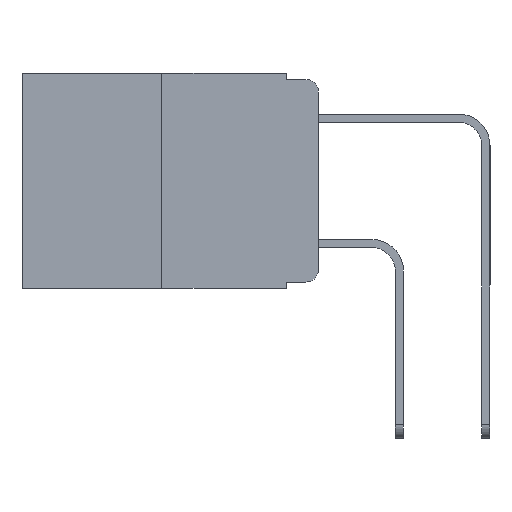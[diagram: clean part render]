
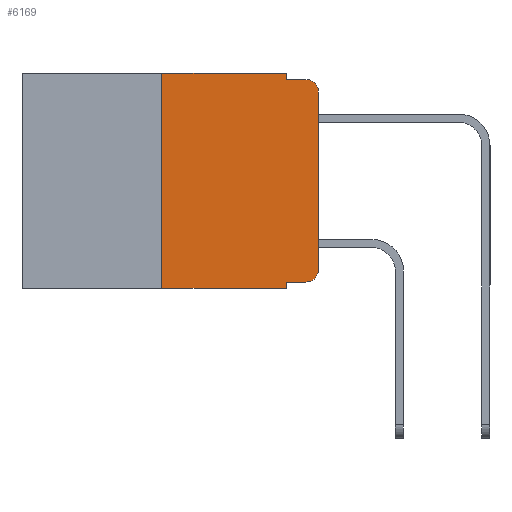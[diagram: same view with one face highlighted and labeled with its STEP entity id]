
A CAD part, left-side view. The second image highlights one B-rep face of the part: STEP entity #6169.
In plain terms, the highlighted planar face has unit normal (-1, 0, 0).
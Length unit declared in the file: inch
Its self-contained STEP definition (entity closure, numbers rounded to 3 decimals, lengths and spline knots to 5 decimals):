
#873 = VECTOR ( 'NONE', #3236, 39.37008 ) ;
#1132 = CARTESIAN_POINT ( 'NONE',  ( 0., 0.02, -0.313 ) ) ;
#1244 = EDGE_CURVE ( 'NONE', #6754, #8812, #8413, .T. ) ;
#1344 = ORIENTED_EDGE ( 'NONE', *, *, #3674, .T. ) ;
#1407 = ORIENTED_EDGE ( 'NONE', *, *, #5270, .T. ) ;
#1428 = ORIENTED_EDGE ( 'NONE', *, *, #2889, .F. ) ;
#1588 = ORIENTED_EDGE ( 'NONE', *, *, #2077, .F. ) ;
#1862 = ORIENTED_EDGE ( 'NONE', *, *, #4581, .F. ) ;
#1973 = ORIENTED_EDGE ( 'NONE', *, *, #1244, .F. ) ;
#2077 = EDGE_CURVE ( 'NONE', #10570, #12774, #9815, .T. ) ;
#2120 = CARTESIAN_POINT ( 'NONE',  ( 0., 0.051, 0. ) ) ;
#2265 = CARTESIAN_POINT ( 'NONE',  ( 0., 0.02, -0.01 ) ) ;
#2370 = DIRECTION ( 'NONE',  ( 0., 0., -1. ) ) ;
#2429 = ORIENTED_EDGE ( 'NONE', *, *, #13222, .T. ) ;
#2438 = VERTEX_POINT ( 'NONE', #2265 ) ;
#2616 = VECTOR ( 'NONE', #14439, 39.37008 ) ;
#2889 = EDGE_CURVE ( 'NONE', #12774, #2438, #8736, .T. ) ;
#3167 = VECTOR ( 'NONE', #14179, 39.37008 ) ;
#3200 = LINE ( 'NONE', #4901, #11684 ) ;
#3236 = DIRECTION ( 'NONE',  ( 0., 0., 1. ) ) ;
#3674 = EDGE_CURVE ( 'NONE', #5236, #2438, #10483, .T. ) ;
#3771 = CARTESIAN_POINT ( 'NONE',  ( 0., 0.051, -0.01 ) ) ;
#4011 = VECTOR ( 'NONE', #12961, 39.37008 ) ;
#4368 = CARTESIAN_POINT ( 'NONE',  ( 0., 0., -0.03 ) ) ;
#4391 = DIRECTION ( 'NONE',  ( 0., -1., 0. ) ) ;
#4423 = CARTESIAN_POINT ( 'NONE',  ( 0., 0., 0. ) ) ;
#4485 = LINE ( 'NONE', #4423, #873 ) ;
#4581 = EDGE_CURVE ( 'NONE', #8812, #10570, #13470, .T. ) ;
#4838 = ORIENTED_EDGE ( 'NONE', *, *, #14728, .F. ) ;
#4901 = CARTESIAN_POINT ( 'NONE',  ( 0., 0.051, -0.333 ) ) ;
#4950 = DIRECTION ( 'NONE',  ( 0., -1., 0. ) ) ;
#5236 = VERTEX_POINT ( 'NONE', #4368 ) ;
#5270 = EDGE_CURVE ( 'NONE', #11873, #5236, #4485, .T. ) ;
#5336 = VECTOR ( 'NONE', #11438, 39.37008 ) ;
#5699 = CARTESIAN_POINT ( 'NONE',  ( 0., 0.02, -0.333 ) ) ;
#5908 = DIRECTION ( 'NONE',  ( -1., 0., 0. ) ) ;
#5923 = CARTESIAN_POINT ( 'NONE',  ( 0., 0.25, 0. ) ) ;
#6169 = ADVANCED_FACE ( 'NONE', ( #7643 ), #13734, .F. ) ;
#6754 = VERTEX_POINT ( 'NONE', #11488 ) ;
#6899 = DIRECTION ( 'NONE',  ( 1., 0., 0. ) ) ;
#7643 = FACE_OUTER_BOUND ( 'NONE', #9121, .T. ) ;
#7682 = VERTEX_POINT ( 'NONE', #11015 ) ;
#7754 = CARTESIAN_POINT ( 'NONE',  ( 0., 0., -0.313 ) ) ;
#7853 = CARTESIAN_POINT ( 'NONE',  ( 0., 0.473, 0. ) ) ;
#8376 = VECTOR ( 'NONE', #14140, 39.37008 ) ;
#8413 = LINE ( 'NONE', #5923, #5336 ) ;
#8556 = CARTESIAN_POINT ( 'NONE',  ( 0., 0.051, 0. ) ) ;
#8736 = LINE ( 'NONE', #3771, #8376 ) ;
#8812 = VERTEX_POINT ( 'NONE', #14089 ) ;
#9121 = EDGE_LOOP ( 'NONE', ( #1407, #1344, #1428, #1588, #1862, #1973, #14688, #4838, #11317, #2429 ) ) ;
#9320 = AXIS2_PLACEMENT_3D ( 'NONE', #10323, #6899, #14877 ) ;
#9359 = LINE ( 'NONE', #8556, #3167 ) ;
#9369 = DIRECTION ( 'NONE',  ( -1., 0., 0. ) ) ;
#9815 = LINE ( 'NONE', #13004, #4011 ) ;
#10111 = VECTOR ( 'NONE', #4391, 39.37008 ) ;
#10323 = CARTESIAN_POINT ( 'NONE',  ( 0., 0.473, 0. ) ) ;
#10483 = CIRCLE ( 'NONE', #13983, 0.02 ) ;
#10570 = VERTEX_POINT ( 'NONE', #2120 ) ;
#10877 = VERTEX_POINT ( 'NONE', #13144 ) ;
#11015 = CARTESIAN_POINT ( 'NONE',  ( 0., 0.051, -0.343 ) ) ;
#11317 = ORIENTED_EDGE ( 'NONE', *, *, #13960, .T. ) ;
#11381 = AXIS2_PLACEMENT_3D ( 'NONE', #1132, #9369, #2370 ) ;
#11438 = DIRECTION ( 'NONE',  ( 0., 0., 1. ) ) ;
#11488 = CARTESIAN_POINT ( 'NONE',  ( 0., 0.25, -0.343 ) ) ;
#11684 = VECTOR ( 'NONE', #4950, 39.37008 ) ;
#11873 = VERTEX_POINT ( 'NONE', #7754 ) ;
#12212 = LINE ( 'NONE', #13313, #2616 ) ;
#12774 = VERTEX_POINT ( 'NONE', #13877 ) ;
#12961 = DIRECTION ( 'NONE',  ( 0., 0., -1. ) ) ;
#13004 = CARTESIAN_POINT ( 'NONE',  ( 0., 0.051, 0. ) ) ;
#13144 = CARTESIAN_POINT ( 'NONE',  ( 0., 0.051, -0.333 ) ) ;
#13157 = VERTEX_POINT ( 'NONE', #5699 ) ;
#13222 = EDGE_CURVE ( 'NONE', #13157, #11873, #13311, .T. ) ;
#13311 = CIRCLE ( 'NONE', #11381, 0.02 ) ;
#13313 = CARTESIAN_POINT ( 'NONE',  ( 0., 0.473, -0.343 ) ) ;
#13470 = LINE ( 'NONE', #7853, #10111 ) ;
#13734 = PLANE ( 'NONE',  #9320 ) ;
#13877 = CARTESIAN_POINT ( 'NONE',  ( 0., 0.051, -0.01 ) ) ;
#13889 = DIRECTION ( 'NONE',  ( 0., 0., -1. ) ) ;
#13960 = EDGE_CURVE ( 'NONE', #10877, #13157, #3200, .T. ) ;
#13983 = AXIS2_PLACEMENT_3D ( 'NONE', #15138, #5908, #13889 ) ;
#14089 = CARTESIAN_POINT ( 'NONE',  ( 0., 0.25, 0. ) ) ;
#14140 = DIRECTION ( 'NONE',  ( 0., -1., 0. ) ) ;
#14148 = EDGE_CURVE ( 'NONE', #6754, #7682, #12212, .T. ) ;
#14179 = DIRECTION ( 'NONE',  ( 0., 0., -1. ) ) ;
#14439 = DIRECTION ( 'NONE',  ( 0., -1., 0. ) ) ;
#14688 = ORIENTED_EDGE ( 'NONE', *, *, #14148, .T. ) ;
#14728 = EDGE_CURVE ( 'NONE', #10877, #7682, #9359, .T. ) ;
#14877 = DIRECTION ( 'NONE',  ( 0., 0., -1. ) ) ;
#15138 = CARTESIAN_POINT ( 'NONE',  ( 0., 0.02, -0.03 ) ) ;
